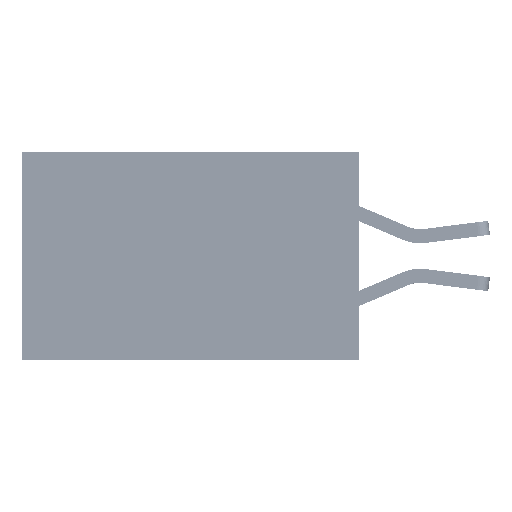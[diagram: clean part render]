
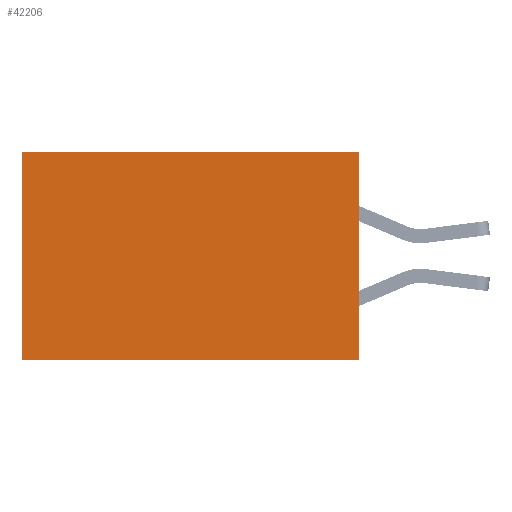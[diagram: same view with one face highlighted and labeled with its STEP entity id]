
A CAD part, left-side view. The second image highlights one B-rep face of the part: STEP entity #42206.
In plain terms, the highlighted planar face has unit normal (-1, 0, 0).
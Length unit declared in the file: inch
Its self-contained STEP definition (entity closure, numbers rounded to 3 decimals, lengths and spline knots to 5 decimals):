
#2726 = EDGE_CURVE ( 'NONE', #27859, #8856, #23766, .T. ) ;
#3223 = EDGE_LOOP ( 'NONE', ( #14386, #23103, #40062, #24845 ) ) ;
#3985 = DIRECTION ( 'NONE',  ( 0., 1., 0. ) ) ;
#4181 = LINE ( 'NONE', #36522, #31947 ) ;
#4490 = CARTESIAN_POINT ( 'NONE',  ( 0.2875, 0., 0. ) ) ;
#7856 = DIRECTION ( 'NONE',  ( 0., 0., -1. ) ) ;
#8765 = FACE_OUTER_BOUND ( 'NONE', #3223, .T. ) ;
#8856 = VERTEX_POINT ( 'NONE', #15239 ) ;
#9116 = EDGE_CURVE ( 'NONE', #15341, #10077, #21551, .T. ) ;
#9326 = DIRECTION ( 'NONE',  ( 0., 0., -1. ) ) ;
#10077 = VERTEX_POINT ( 'NONE', #40199 ) ;
#12329 = VECTOR ( 'NONE', #40472, 39.37008 ) ;
#13381 = EDGE_CURVE ( 'NONE', #10077, #8856, #4181, .T. ) ;
#14386 = ORIENTED_EDGE ( 'NONE', *, *, #2726, .T. ) ;
#15239 = CARTESIAN_POINT ( 'NONE',  ( 0.2875, 0.6, -0.37 ) ) ;
#15341 = VERTEX_POINT ( 'NONE', #21969 ) ;
#18865 = EDGE_CURVE ( 'NONE', #15341, #27859, #39986, .T. ) ;
#21018 = CARTESIAN_POINT ( 'NONE',  ( 0.2875, 0.6, 0. ) ) ;
#21551 = LINE ( 'NONE', #38063, #39555 ) ;
#21969 = CARTESIAN_POINT ( 'NONE',  ( 0.2875, 0., 0. ) ) ;
#22559 = AXIS2_PLACEMENT_3D ( 'NONE', #25933, #29561, #7856 ) ;
#23103 = ORIENTED_EDGE ( 'NONE', *, *, #13381, .F. ) ;
#23766 = LINE ( 'NONE', #40088, #41743 ) ;
#24845 = ORIENTED_EDGE ( 'NONE', *, *, #18865, .T. ) ;
#25933 = CARTESIAN_POINT ( 'NONE',  ( 0.2875, 0., 0. ) ) ;
#27859 = VERTEX_POINT ( 'NONE', #21018 ) ;
#29561 = DIRECTION ( 'NONE',  ( 1., 0., 0. ) ) ;
#31947 = VECTOR ( 'NONE', #3985, 39.37008 ) ;
#36522 = CARTESIAN_POINT ( 'NONE',  ( 0.2875, 0., -0.37 ) ) ;
#36794 = DIRECTION ( 'NONE',  ( 0., 0., -1. ) ) ;
#38063 = CARTESIAN_POINT ( 'NONE',  ( 0.2875, 0., 0. ) ) ;
#39555 = VECTOR ( 'NONE', #9326, 39.37008 ) ;
#39986 = LINE ( 'NONE', #4490, #12329 ) ;
#40062 = ORIENTED_EDGE ( 'NONE', *, *, #9116, .F. ) ;
#40088 = CARTESIAN_POINT ( 'NONE',  ( 0.2875, 0.6, 0. ) ) ;
#40199 = CARTESIAN_POINT ( 'NONE',  ( 0.2875, 0., -0.37 ) ) ;
#40212 = PLANE ( 'NONE',  #22559 ) ;
#40472 = DIRECTION ( 'NONE',  ( 0., 1., 0. ) ) ;
#41743 = VECTOR ( 'NONE', #36794, 39.37008 ) ;
#42206 = ADVANCED_FACE ( 'NONE', ( #8765 ), #40212, .F. ) ;
